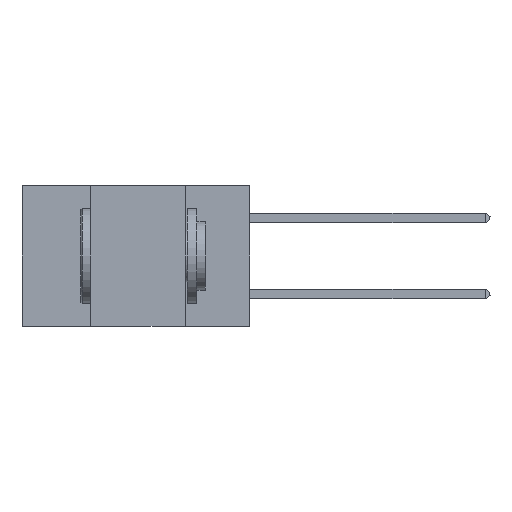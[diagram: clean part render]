
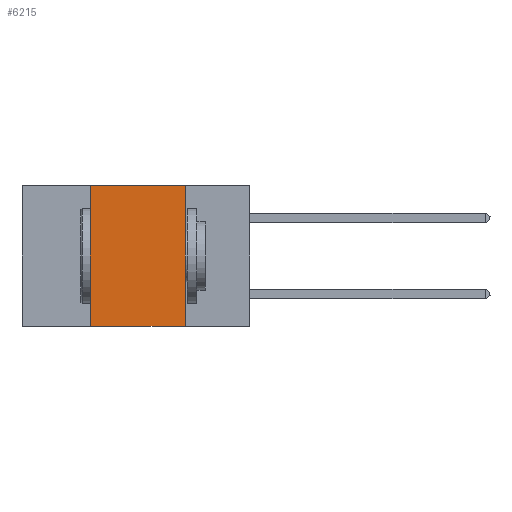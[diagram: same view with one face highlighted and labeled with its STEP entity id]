
A CAD part, left-side view. The second image highlights one B-rep face of the part: STEP entity #6215.
In plain terms, the highlighted planar face has unit normal (-1, 0, 0).
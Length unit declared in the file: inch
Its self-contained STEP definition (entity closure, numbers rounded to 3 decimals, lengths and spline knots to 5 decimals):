
#462 = DIRECTION ( 'NONE',  ( 0., -1., 0. ) ) ;
#916 = DIRECTION ( 'NONE',  ( 0., -1., 0. ) ) ;
#1005 = VECTOR ( 'NONE', #6319, 39.37008 ) ;
#1017 = VECTOR ( 'NONE', #1789, 39.37008 ) ;
#1789 = DIRECTION ( 'NONE',  ( 0., 0., 1. ) ) ;
#1931 = AXIS2_PLACEMENT_3D ( 'NONE', #2035, #9238, #4002 ) ;
#2006 = EDGE_CURVE ( 'NONE', #2186, #4884, #8337, .T. ) ;
#2035 = CARTESIAN_POINT ( 'NONE',  ( 0., 0.6, 0. ) ) ;
#2186 = VERTEX_POINT ( 'NONE', #2264 ) ;
#2264 = CARTESIAN_POINT ( 'NONE',  ( 0., 0.17, 0. ) ) ;
#2936 = FACE_OUTER_BOUND ( 'NONE', #10289, .T. ) ;
#3646 = LINE ( 'NONE', #9851, #1017 ) ;
#3755 = CARTESIAN_POINT ( 'NONE',  ( 0., 0.42, 0. ) ) ;
#3773 = ORIENTED_EDGE ( 'NONE', *, *, #2006, .F. ) ;
#4002 = DIRECTION ( 'NONE',  ( 0., 0., -1. ) ) ;
#4884 = VERTEX_POINT ( 'NONE', #7782 ) ;
#6058 = VECTOR ( 'NONE', #462, 39.37008 ) ;
#6215 = ADVANCED_FACE ( 'NONE', ( #2936 ), #8380, .F. ) ;
#6238 = LINE ( 'NONE', #6561, #10805 ) ;
#6267 = CARTESIAN_POINT ( 'NONE',  ( 0., 0.17, 0. ) ) ;
#6319 = DIRECTION ( 'NONE',  ( 0., 0., -1. ) ) ;
#6561 = CARTESIAN_POINT ( 'NONE',  ( 0., 0.6, -0.37 ) ) ;
#6721 = ORIENTED_EDGE ( 'NONE', *, *, #8535, .F. ) ;
#6987 = CARTESIAN_POINT ( 'NONE',  ( 0., 0.42, -0.37 ) ) ;
#7681 = EDGE_CURVE ( 'NONE', #8524, #2186, #10637, .T. ) ;
#7782 = CARTESIAN_POINT ( 'NONE',  ( 0., 0.17, -0.37 ) ) ;
#8337 = LINE ( 'NONE', #6267, #1005 ) ;
#8380 = PLANE ( 'NONE',  #1931 ) ;
#8524 = VERTEX_POINT ( 'NONE', #3755 ) ;
#8535 = EDGE_CURVE ( 'NONE', #11331, #8524, #3646, .T. ) ;
#9238 = DIRECTION ( 'NONE',  ( 1., 0., 0. ) ) ;
#9811 = EDGE_CURVE ( 'NONE', #11331, #4884, #6238, .T. ) ;
#9851 = CARTESIAN_POINT ( 'NONE',  ( 0., 0.42, 0. ) ) ;
#10289 = EDGE_LOOP ( 'NONE', ( #3773, #10994, #6721, #11278 ) ) ;
#10637 = LINE ( 'NONE', #11284, #6058 ) ;
#10805 = VECTOR ( 'NONE', #916, 39.37008 ) ;
#10994 = ORIENTED_EDGE ( 'NONE', *, *, #7681, .F. ) ;
#11278 = ORIENTED_EDGE ( 'NONE', *, *, #9811, .T. ) ;
#11284 = CARTESIAN_POINT ( 'NONE',  ( 0., 0.6, 0. ) ) ;
#11331 = VERTEX_POINT ( 'NONE', #6987 ) ;
